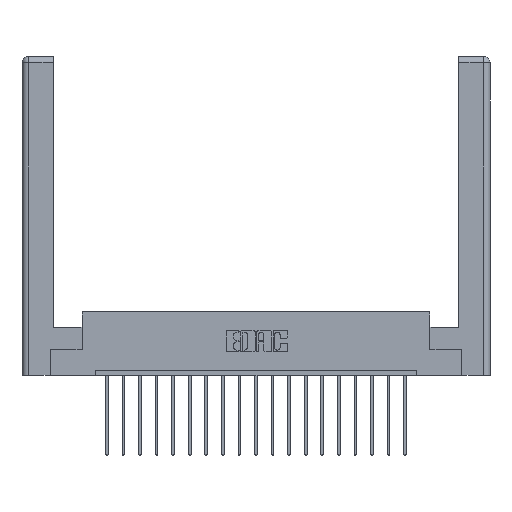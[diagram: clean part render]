
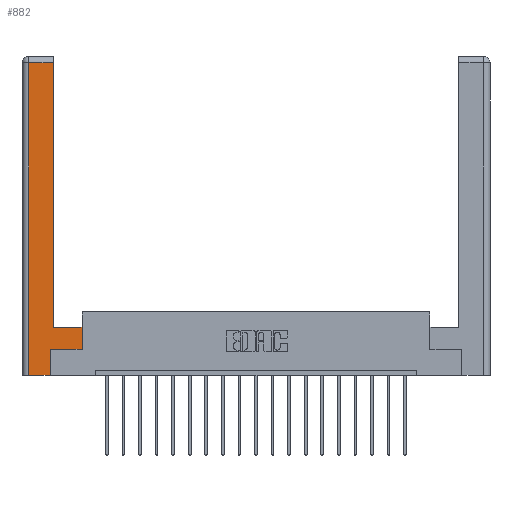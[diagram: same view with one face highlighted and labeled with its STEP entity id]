
A CAD part, top view. The second image highlights one B-rep face of the part: STEP entity #882.
In plain terms, the highlighted planar face has unit normal (0, 0, 1).
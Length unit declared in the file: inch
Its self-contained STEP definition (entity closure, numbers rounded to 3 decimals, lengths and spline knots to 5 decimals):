
#812 = VECTOR ( 'NONE', #1750, 39.37008 ) ;
#882 = ADVANCED_FACE ( 'NONE', ( #9405 ), #14869, .F. ) ;
#1097 = DIRECTION ( 'NONE',  ( -1., 0., 0. ) ) ;
#1173 = CARTESIAN_POINT ( 'NONE',  ( 0.565, 0.45, 0. ) ) ;
#1336 = VECTOR ( 'NONE', #8249, 39.37008 ) ;
#1344 = EDGE_CURVE ( 'NONE', #6762, #9219, #13187, .T. ) ;
#1750 = DIRECTION ( 'NONE',  ( 0., 1., 0. ) ) ;
#1964 = VERTEX_POINT ( 'NONE', #18808 ) ;
#2684 = CARTESIAN_POINT ( 'NONE',  ( 0., 0., 0. ) ) ;
#2748 = CARTESIAN_POINT ( 'NONE',  ( 0.295, 2.94, 0. ) ) ;
#2880 = LINE ( 'NONE', #7824, #10032 ) ;
#3165 = DIRECTION ( 'NONE',  ( 0., -1., 0. ) ) ;
#4050 = ORIENTED_EDGE ( 'NONE', *, *, #6356, .T. ) ;
#4362 = DIRECTION ( 'NONE',  ( 0., 0., -1. ) ) ;
#4617 = EDGE_CURVE ( 'NONE', #14611, #15559, #9132, .T. ) ;
#4626 = VECTOR ( 'NONE', #8415, 39.37008 ) ;
#5201 = DIRECTION ( 'NONE',  ( 1., 0., 0. ) ) ;
#5422 = LINE ( 'NONE', #10024, #1336 ) ;
#5503 = VERTEX_POINT ( 'NONE', #18699 ) ;
#5504 = AXIS2_PLACEMENT_3D ( 'NONE', #2684, #4362, #1097 ) ;
#5565 = ORIENTED_EDGE ( 'NONE', *, *, #8067, .T. ) ;
#5828 = VECTOR ( 'NONE', #3165, 39.37008 ) ;
#6356 = EDGE_CURVE ( 'NONE', #7375, #6762, #6907, .T. ) ;
#6498 = ORIENTED_EDGE ( 'NONE', *, *, #10933, .T. ) ;
#6718 = DIRECTION ( 'NONE',  ( -1., 0., 0. ) ) ;
#6762 = VERTEX_POINT ( 'NONE', #18400 ) ;
#6907 = LINE ( 'NONE', #12686, #12600 ) ;
#7110 = ORIENTED_EDGE ( 'NONE', *, *, #18424, .T. ) ;
#7375 = VERTEX_POINT ( 'NONE', #1173 ) ;
#7703 = CARTESIAN_POINT ( 'NONE',  ( 0.565, 0.245, 0. ) ) ;
#7824 = CARTESIAN_POINT ( 'NONE',  ( 0.0615, 2.94, 0. ) ) ;
#8026 = EDGE_CURVE ( 'NONE', #5503, #13295, #15418, .T. ) ;
#8067 = EDGE_CURVE ( 'NONE', #13295, #7375, #5422, .T. ) ;
#8249 = DIRECTION ( 'NONE',  ( 0., 1., 0. ) ) ;
#8415 = DIRECTION ( 'NONE',  ( 0., 1., 0. ) ) ;
#9034 = EDGE_CURVE ( 'NONE', #15559, #1964, #14246, .T. ) ;
#9132 = LINE ( 'NONE', #13696, #5828 ) ;
#9219 = VERTEX_POINT ( 'NONE', #2748 ) ;
#9239 = ORIENTED_EDGE ( 'NONE', *, *, #4617, .T. ) ;
#9292 = CARTESIAN_POINT ( 'NONE',  ( 0.0615, 0., 0. ) ) ;
#9405 = FACE_OUTER_BOUND ( 'NONE', #11550, .T. ) ;
#10024 = CARTESIAN_POINT ( 'NONE',  ( 0.565, 0.45, 0. ) ) ;
#10032 = VECTOR ( 'NONE', #13864, 39.37008 ) ;
#10933 = EDGE_CURVE ( 'NONE', #1964, #5503, #15359, .T. ) ;
#11148 = VECTOR ( 'NONE', #13198, 39.37008 ) ;
#11203 = CARTESIAN_POINT ( 'NONE',  ( 0.0615, 2.94, 0. ) ) ;
#11293 = ORIENTED_EDGE ( 'NONE', *, *, #9034, .T. ) ;
#11550 = EDGE_LOOP ( 'NONE', ( #14360, #7110, #9239, #11293, #6498, #13381, #5565, #4050 ) ) ;
#12600 = VECTOR ( 'NONE', #6718, 39.37008 ) ;
#12686 = CARTESIAN_POINT ( 'NONE',  ( 0.295, 0.45, 0. ) ) ;
#13187 = LINE ( 'NONE', #14542, #4626 ) ;
#13198 = DIRECTION ( 'NONE',  ( 1., 0., 0. ) ) ;
#13295 = VERTEX_POINT ( 'NONE', #7703 ) ;
#13381 = ORIENTED_EDGE ( 'NONE', *, *, #8026, .T. ) ;
#13696 = CARTESIAN_POINT ( 'NONE',  ( 0.0615, 0., 0. ) ) ;
#13864 = DIRECTION ( 'NONE',  ( -1., 0., 0. ) ) ;
#14246 = LINE ( 'NONE', #16372, #11148 ) ;
#14360 = ORIENTED_EDGE ( 'NONE', *, *, #1344, .T. ) ;
#14542 = CARTESIAN_POINT ( 'NONE',  ( 0.295, 3., 0. ) ) ;
#14611 = VERTEX_POINT ( 'NONE', #11203 ) ;
#14869 = PLANE ( 'NONE',  #5504 ) ;
#15359 = LINE ( 'NONE', #18684, #812 ) ;
#15418 = LINE ( 'NONE', #17605, #17578 ) ;
#15559 = VERTEX_POINT ( 'NONE', #9292 ) ;
#16372 = CARTESIAN_POINT ( 'NONE',  ( 0.265, 0., 0. ) ) ;
#17578 = VECTOR ( 'NONE', #5201, 39.37008 ) ;
#17605 = CARTESIAN_POINT ( 'NONE',  ( 0.565, 0.245, 0. ) ) ;
#18400 = CARTESIAN_POINT ( 'NONE',  ( 0.295, 0.45, 0. ) ) ;
#18424 = EDGE_CURVE ( 'NONE', #9219, #14611, #2880, .T. ) ;
#18684 = CARTESIAN_POINT ( 'NONE',  ( 0.265, 0.245, 0. ) ) ;
#18699 = CARTESIAN_POINT ( 'NONE',  ( 0.265, 0.245, 0. ) ) ;
#18808 = CARTESIAN_POINT ( 'NONE',  ( 0.265, 0., 0. ) ) ;
